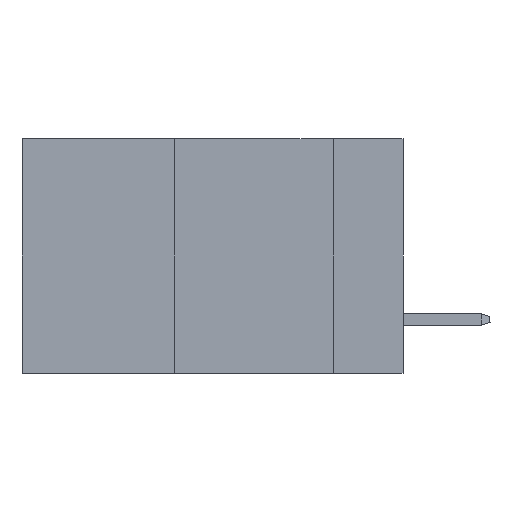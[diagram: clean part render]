
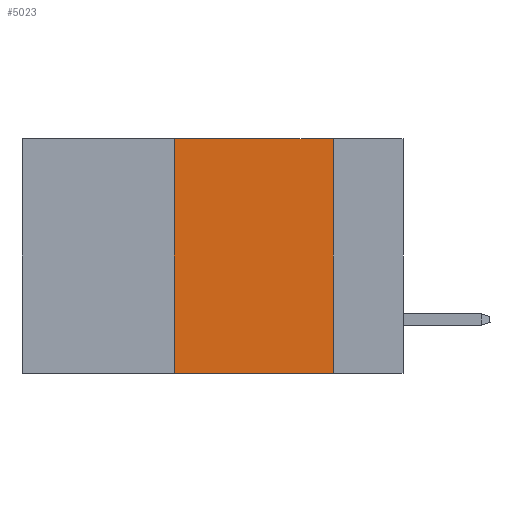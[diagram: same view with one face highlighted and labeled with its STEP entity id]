
A CAD part, left-side view. The second image highlights one B-rep face of the part: STEP entity #5023.
In plain terms, the highlighted planar face has unit normal (-1, 0, 0).
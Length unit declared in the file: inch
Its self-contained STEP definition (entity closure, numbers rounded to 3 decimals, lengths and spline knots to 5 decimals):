
#1069 = CARTESIAN_POINT ( 'NONE',  ( 0., 0.6, -0.37 ) ) ;
#2220 = FACE_OUTER_BOUND ( 'NONE', #23868, .T. ) ;
#2620 = VECTOR ( 'NONE', #16481, 39.37008 ) ;
#2676 = LINE ( 'NONE', #17145, #2620 ) ;
#4032 = VERTEX_POINT ( 'NONE', #18031 ) ;
#4639 = LINE ( 'NONE', #15502, #40764 ) ;
#5023 = ADVANCED_FACE ( 'NONE', ( #2220 ), #30082, .F. ) ;
#9737 = VERTEX_POINT ( 'NONE', #26932 ) ;
#12151 = DIRECTION ( 'NONE',  ( 0., -1., 0. ) ) ;
#12213 = EDGE_CURVE ( 'NONE', #41949, #9737, #4639, .T. ) ;
#12481 = AXIS2_PLACEMENT_3D ( 'NONE', #26666, #15803, #40523 ) ;
#12863 = LINE ( 'NONE', #23037, #35169 ) ;
#14231 = ORIENTED_EDGE ( 'NONE', *, *, #19756, .F. ) ;
#15502 = CARTESIAN_POINT ( 'NONE',  ( 0., 0.36, 0. ) ) ;
#15803 = DIRECTION ( 'NONE',  ( 1., 0., 0. ) ) ;
#15987 = EDGE_CURVE ( 'NONE', #9737, #25768, #2676, .T. ) ;
#16481 = DIRECTION ( 'NONE',  ( 0., -1., 0. ) ) ;
#16785 = ORIENTED_EDGE ( 'NONE', *, *, #12213, .F. ) ;
#17145 = CARTESIAN_POINT ( 'NONE',  ( 0., 0.6, 0. ) ) ;
#18031 = CARTESIAN_POINT ( 'NONE',  ( 0., 0.11, -0.37 ) ) ;
#18711 = ORIENTED_EDGE ( 'NONE', *, *, #15987, .F. ) ;
#19756 = EDGE_CURVE ( 'NONE', #25768, #4032, #12863, .T. ) ;
#19933 = CARTESIAN_POINT ( 'NONE',  ( 0., 0.36, -0.37 ) ) ;
#21380 = EDGE_CURVE ( 'NONE', #41949, #4032, #22319, .T. ) ;
#21929 = ORIENTED_EDGE ( 'NONE', *, *, #21380, .T. ) ;
#22278 = DIRECTION ( 'NONE',  ( 0., 0., 1. ) ) ;
#22319 = LINE ( 'NONE', #1069, #35788 ) ;
#23037 = CARTESIAN_POINT ( 'NONE',  ( 0., 0.11, 0. ) ) ;
#23868 = EDGE_LOOP ( 'NONE', ( #14231, #18711, #16785, #21929 ) ) ;
#24384 = CARTESIAN_POINT ( 'NONE',  ( 0., 0.11, 0. ) ) ;
#25768 = VERTEX_POINT ( 'NONE', #24384 ) ;
#26453 = DIRECTION ( 'NONE',  ( 0., 0., -1. ) ) ;
#26666 = CARTESIAN_POINT ( 'NONE',  ( 0., 0.6, 0. ) ) ;
#26932 = CARTESIAN_POINT ( 'NONE',  ( 0., 0.36, 0. ) ) ;
#30082 = PLANE ( 'NONE',  #12481 ) ;
#35169 = VECTOR ( 'NONE', #26453, 39.37008 ) ;
#35788 = VECTOR ( 'NONE', #12151, 39.37008 ) ;
#40523 = DIRECTION ( 'NONE',  ( 0., 0., -1. ) ) ;
#40764 = VECTOR ( 'NONE', #22278, 39.37008 ) ;
#41949 = VERTEX_POINT ( 'NONE', #19933 ) ;
